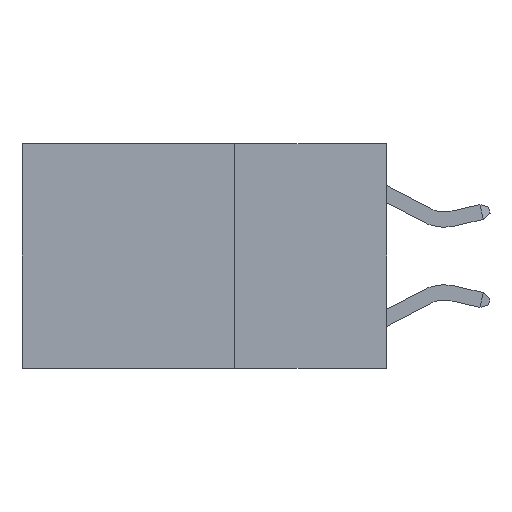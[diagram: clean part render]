
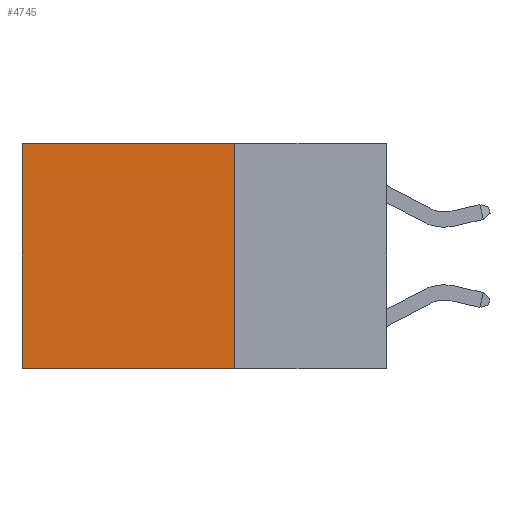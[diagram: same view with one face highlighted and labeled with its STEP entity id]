
A CAD part, left-side view. The second image highlights one B-rep face of the part: STEP entity #4745.
In plain terms, the highlighted planar face has unit normal (-1, 0, 0).
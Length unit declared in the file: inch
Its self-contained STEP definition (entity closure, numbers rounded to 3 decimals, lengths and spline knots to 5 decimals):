
#246 = LINE ( 'NONE', #3154, #13402 ) ;
#279 = ORIENTED_EDGE ( 'NONE', *, *, #10068, .F. ) ;
#369 = ORIENTED_EDGE ( 'NONE', *, *, #1093, .T. ) ;
#1093 = EDGE_CURVE ( 'NONE', #10428, #9813, #246, .T. ) ;
#1725 = CARTESIAN_POINT ( 'NONE',  ( 0.2625, 0.25, 0. ) ) ;
#1973 = DIRECTION ( 'NONE',  ( 0., 1., 0. ) ) ;
#2101 = VECTOR ( 'NONE', #5528, 39.37008 ) ;
#2191 = CARTESIAN_POINT ( 'NONE',  ( 0.2625, 0.6, 0. ) ) ;
#2837 = DIRECTION ( 'NONE',  ( 0., 1., 0. ) ) ;
#2852 = DIRECTION ( 'NONE',  ( 0., 0., -1. ) ) ;
#3154 = CARTESIAN_POINT ( 'NONE',  ( 0.2625, 0.25, 0. ) ) ;
#3696 = VECTOR ( 'NONE', #12721, 39.37008 ) ;
#3781 = PLANE ( 'NONE',  #6966 ) ;
#4745 = ADVANCED_FACE ( 'NONE', ( #11632 ), #3781, .F. ) ;
#4990 = EDGE_CURVE ( 'NONE', #9813, #10324, #13002, .T. ) ;
#5262 = LINE ( 'NONE', #6562, #3696 ) ;
#5528 = DIRECTION ( 'NONE',  ( 0., 0., -1. ) ) ;
#5693 = CARTESIAN_POINT ( 'NONE',  ( 0.2625, 0.25, -0.37 ) ) ;
#6342 = CARTESIAN_POINT ( 'NONE',  ( 0.2625, 0.25, 0. ) ) ;
#6562 = CARTESIAN_POINT ( 'NONE',  ( 0.2625, 0.25, 0. ) ) ;
#6894 = LINE ( 'NONE', #8233, #7397 ) ;
#6920 = VERTEX_POINT ( 'NONE', #5693 ) ;
#6966 = AXIS2_PLACEMENT_3D ( 'NONE', #1725, #7095, #2852 ) ;
#7095 = DIRECTION ( 'NONE',  ( 1., 0., 0. ) ) ;
#7397 = VECTOR ( 'NONE', #2837, 39.37008 ) ;
#7569 = ORIENTED_EDGE ( 'NONE', *, *, #13912, .F. ) ;
#8233 = CARTESIAN_POINT ( 'NONE',  ( 0.2625, 0.25, -0.37 ) ) ;
#9298 = ORIENTED_EDGE ( 'NONE', *, *, #4990, .T. ) ;
#9813 = VERTEX_POINT ( 'NONE', #10981 ) ;
#10068 = EDGE_CURVE ( 'NONE', #10428, #6920, #5262, .T. ) ;
#10324 = VERTEX_POINT ( 'NONE', #13653 ) ;
#10428 = VERTEX_POINT ( 'NONE', #6342 ) ;
#10946 = EDGE_LOOP ( 'NONE', ( #9298, #7569, #279, #369 ) ) ;
#10981 = CARTESIAN_POINT ( 'NONE',  ( 0.2625, 0.6, 0. ) ) ;
#11632 = FACE_OUTER_BOUND ( 'NONE', #10946, .T. ) ;
#12721 = DIRECTION ( 'NONE',  ( 0., 0., -1. ) ) ;
#13002 = LINE ( 'NONE', #2191, #2101 ) ;
#13402 = VECTOR ( 'NONE', #1973, 39.37008 ) ;
#13653 = CARTESIAN_POINT ( 'NONE',  ( 0.2625, 0.6, -0.37 ) ) ;
#13912 = EDGE_CURVE ( 'NONE', #6920, #10324, #6894, .T. ) ;
